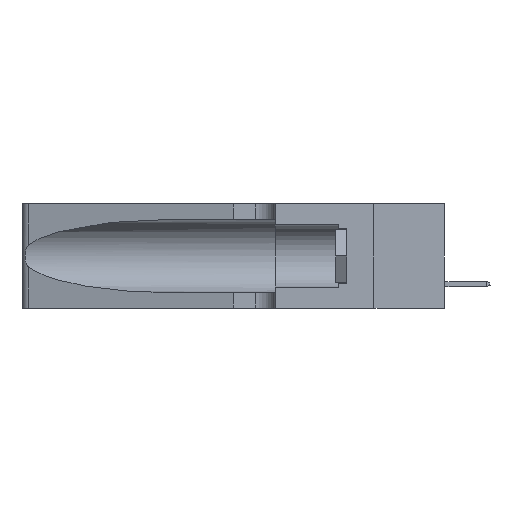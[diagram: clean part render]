
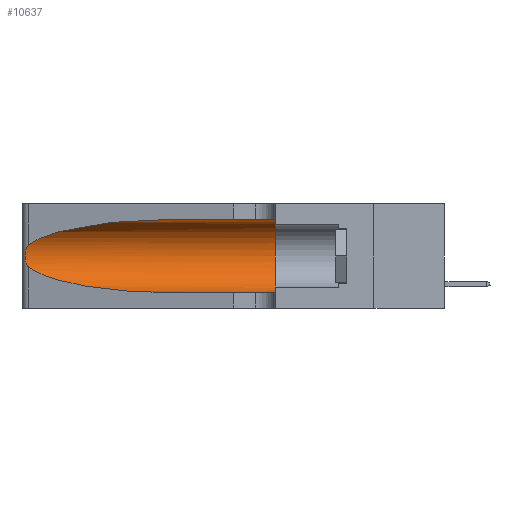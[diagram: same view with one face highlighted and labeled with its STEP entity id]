
A CAD part, left-side view. The second image highlights one B-rep face of the part: STEP entity #10637.
In plain terms, the highlighted cylindrical face has radius 3.308 mm (diameter 6.617 mm), a partial arc.
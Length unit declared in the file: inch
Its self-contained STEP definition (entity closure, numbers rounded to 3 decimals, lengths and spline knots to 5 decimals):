
#1827 = ORIENTED_EDGE ( 'NONE', *, *, #32436, .T. ) ;
#1994 = CARTESIAN_POINT ( 'NONE',  ( 0.18966, 0.96281, 0.31525 ) ) ;
#2345 = EDGE_LOOP ( 'NONE', ( #1827, #20203, #28351, #45309, #46828, #22798 ) ) ;
#2590 = CARTESIAN_POINT ( 'NONE',  ( 0.25856, 1.23593, 0.16098 ) ) ;
#2861 = EDGE_CURVE ( 'NONE', #12255, #17981, #20788, .T. ) ;
#2938 = CARTESIAN_POINT ( 'NONE',  ( 0.25555, 1.22993, 0.14849 ) ) ;
#3188 = EDGE_CURVE ( 'NONE', #22796, #12255, #19856, .T. ) ;
#3799 = CARTESIAN_POINT ( 'NONE',  ( 0.1305, 0.72297, 0.31525 ) ) ;
#4464 = CARTESIAN_POINT ( 'NONE',  ( 0.2373, 1.15595, 0.08982 ) ) ;
#6404 = CARTESIAN_POINT ( 'NONE',  ( 0.26018, 1.23835, 0.19895 ) ) ;
#7401 = CARTESIAN_POINT ( 'NONE',  ( 0.1305, 1.61858, 0.185 ) ) ;
#8440 = CARTESIAN_POINT ( 'NONE',  ( 0.1305, 0.72297, 0.05475 ) ) ;
#9785 = CARTESIAN_POINT ( 'NONE',  ( 0.25487, 1.22718, 0.22369 ) ) ;
#10627 = DIRECTION ( 'NONE',  ( 0., 0., 1. ) ) ;
#10637 = ADVANCED_FACE ( 'NONE', ( #15573 ), #39013, .F. ) ;
#10744 = CARTESIAN_POINT ( 'NONE',  ( 0.26075, 1.23896, 0.178 ) ) ;
#10796 = DIRECTION ( 'NONE',  ( 0., 1., 0. ) ) ;
#11256 = CARTESIAN_POINT ( 'NONE',  ( 0.1305, 1.61858, 0.05475 ) ) ;
#11731 = DIRECTION ( 'NONE',  ( 0., 0., -1. ) ) ;
#12255 = VERTEX_POINT ( 'NONE', #28409 ) ;
#12988 = CARTESIAN_POINT ( 'NONE',  ( 0.25487, 1.22718, 0.22369 ) ) ;
#13669 = CARTESIAN_POINT ( 'NONE',  ( 0.25787, 1.23484, 0.2124 ) ) ;
#14026 = CARTESIAN_POINT ( 'NONE',  ( 0.25487, 1.22718, 0.14631 ) ) ;
#14208 = CARTESIAN_POINT ( 'NONE',  ( 0.25854, 1.2359, 0.20912 ) ) ;
#14475 = LINE ( 'NONE', #11256, #47752 ) ;
#14496 = EDGE_CURVE ( 'NONE', #27393, #33548, #46538, .T. ) ;
#15573 = FACE_OUTER_BOUND ( 'NONE', #2345, .T. ) ;
#17981 = VERTEX_POINT ( 'NONE', #23370 ) ;
#18860 = DIRECTION ( 'NONE',  ( 0., -1., 0. ) ) ;
#19652 = DIRECTION ( 'NONE',  ( 0., -1., 0. ) ) ;
#19856 = B_SPLINE_CURVE_WITH_KNOTS ( 'NONE', 3,
 ( #12988, #21448, #25089, #13669, #14208, #6404, #37646, #10744, #34049, #2590, #22537, #30304, #2938, #14026 ),
 .UNSPECIFIED., .F., .F.,
 ( 4, 2, 2, 2, 2, 2, 4 ),
 ( 0., 0.00027, 0.00053, 0.00107, 0.0016, 0.00187, 0.00214 ),
 .UNSPECIFIED. ) ;
#20203 = ORIENTED_EDGE ( 'NONE', *, *, #3188, .T. ) ;
#20788 =( BOUNDED_CURVE ( )  B_SPLINE_CURVE ( 3, ( #28154, #4464, #48455, #8440 ),
 .UNSPECIFIED., .F., .T. ) 
 B_SPLINE_CURVE_WITH_KNOTS ( ( 4, 4 ),
 ( 3.44316, 4.71239 ),
 .UNSPECIFIED. ) 
 CURVE ( )  GEOMETRIC_REPRESENTATION_ITEM ( )  RATIONAL_B_SPLINE_CURVE ( ( 1., 0.87, 0.87, 1. ) ) 
 REPRESENTATION_ITEM ( '' )  );
#21324 = CARTESIAN_POINT ( 'NONE',  ( 0.25487, 1.22718, 0.22369 ) ) ;
#21448 = CARTESIAN_POINT ( 'NONE',  ( 0.25555, 1.22994, 0.2215 ) ) ;
#22537 = CARTESIAN_POINT ( 'NONE',  ( 0.25789, 1.23486, 0.15765 ) ) ;
#22796 = VERTEX_POINT ( 'NONE', #21324 ) ;
#22798 = ORIENTED_EDGE ( 'NONE', *, *, #14496, .F. ) ;
#22939 = CARTESIAN_POINT ( 'NONE',  ( 0.1305, 0.35, 0.31525 ) ) ;
#23370 = CARTESIAN_POINT ( 'NONE',  ( 0.1305, 0.72297, 0.05475 ) ) ;
#25089 = CARTESIAN_POINT ( 'NONE',  ( 0.25639, 1.23184, 0.21858 ) ) ;
#27390 = CARTESIAN_POINT ( 'NONE',  ( 0.1305, 0.35, 0.05475 ) ) ;
#27393 = VERTEX_POINT ( 'NONE', #3799 ) ;
#27895 = DIRECTION ( 'NONE',  ( 0., -1., 0. ) ) ;
#28154 = CARTESIAN_POINT ( 'NONE',  ( 0.25487, 1.22718, 0.14631 ) ) ;
#28351 = ORIENTED_EDGE ( 'NONE', *, *, #2861, .T. ) ;
#28409 = CARTESIAN_POINT ( 'NONE',  ( 0.25487, 1.22718, 0.14631 ) ) ;
#29663 = EDGE_CURVE ( 'NONE', #17981, #48133, #14475, .T. ) ;
#30304 = CARTESIAN_POINT ( 'NONE',  ( 0.25639, 1.23186, 0.15144 ) ) ;
#32436 = EDGE_CURVE ( 'NONE', #27393, #22796, #48924, .T. ) ;
#33111 = CARTESIAN_POINT ( 'NONE',  ( 0.2373, 1.15595, 0.28018 ) ) ;
#33548 = VERTEX_POINT ( 'NONE', #22939 ) ;
#34049 = CARTESIAN_POINT ( 'NONE',  ( 0.26017, 1.23833, 0.17102 ) ) ;
#34459 = CARTESIAN_POINT ( 'NONE',  ( 0.1305, 0.35, 0.185 ) ) ;
#37364 = AXIS2_PLACEMENT_3D ( 'NONE', #7401, #19652, #11731 ) ;
#37646 = CARTESIAN_POINT ( 'NONE',  ( 0.26075, 1.23896, 0.19203 ) ) ;
#39013 = CYLINDRICAL_SURFACE ( 'NONE', #37364, 0.13025 ) ;
#39869 = AXIS2_PLACEMENT_3D ( 'NONE', #34459, #10796, #10627 ) ;
#41663 = EDGE_CURVE ( 'NONE', #33548, #48133, #49833, .T. ) ;
#44584 = CARTESIAN_POINT ( 'NONE',  ( 0.1305, 1.61858, 0.31525 ) ) ;
#45309 = ORIENTED_EDGE ( 'NONE', *, *, #29663, .T. ) ;
#46538 = LINE ( 'NONE', #44584, #49636 ) ;
#46828 = ORIENTED_EDGE ( 'NONE', *, *, #41663, .F. ) ;
#47752 = VECTOR ( 'NONE', #18860, 39.37008 ) ;
#48133 = VERTEX_POINT ( 'NONE', #27390 ) ;
#48455 = CARTESIAN_POINT ( 'NONE',  ( 0.18966, 0.96281, 0.05475 ) ) ;
#48924 =( BOUNDED_CURVE ( )  B_SPLINE_CURVE ( 3, ( #48960, #1994, #33111, #9785 ),
 .UNSPECIFIED., .F., .F. ) 
 B_SPLINE_CURVE_WITH_KNOTS ( ( 4, 4 ),
 ( 1.5708, 2.84003 ),
 .UNSPECIFIED. ) 
 CURVE ( )  GEOMETRIC_REPRESENTATION_ITEM ( )  RATIONAL_B_SPLINE_CURVE ( ( 1., 0.87, 0.87, 1. ) ) 
 REPRESENTATION_ITEM ( '' )  );
#48960 = CARTESIAN_POINT ( 'NONE',  ( 0.1305, 0.72297, 0.31525 ) ) ;
#49636 = VECTOR ( 'NONE', #27895, 39.37008 ) ;
#49833 = CIRCLE ( 'NONE', #39869, 0.13025 ) ;
